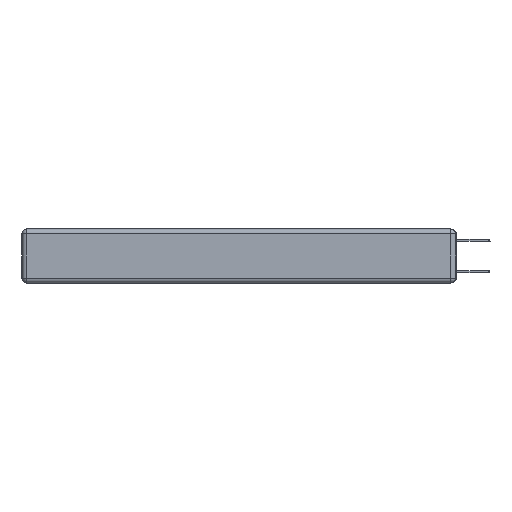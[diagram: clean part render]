
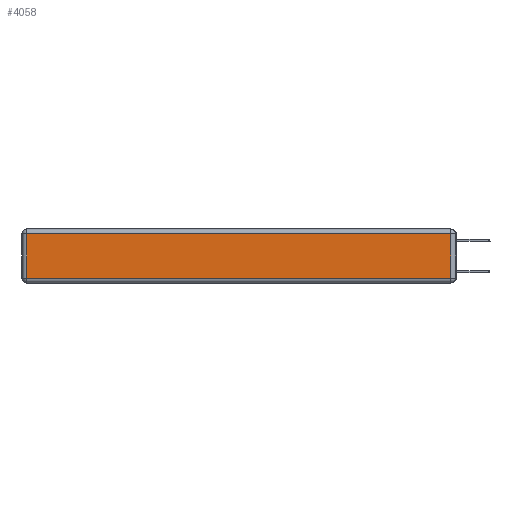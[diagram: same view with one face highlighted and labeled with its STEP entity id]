
A CAD part, left-side view. The second image highlights one B-rep face of the part: STEP entity #4058.
In plain terms, the highlighted planar face has unit normal (-1, 0, 0).
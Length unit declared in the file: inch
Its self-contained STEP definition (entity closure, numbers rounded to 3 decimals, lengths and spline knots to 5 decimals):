
#633 = VERTEX_POINT ( 'NONE', #15095 ) ;
#755 = PLANE ( 'NONE',  #25407 ) ;
#1755 = VERTEX_POINT ( 'NONE', #6588 ) ;
#2178 = ORIENTED_EDGE ( 'NONE', *, *, #19815, .T. ) ;
#2660 = EDGE_CURVE ( 'NONE', #22898, #25426, #4708, .T. ) ;
#3557 = VECTOR ( 'NONE', #8804, 39.37008 ) ;
#4058 = ADVANCED_FACE ( 'NONE', ( #20680 ), #755, .T. ) ;
#4284 = CARTESIAN_POINT ( 'NONE',  ( 0., 0., -0.343 ) ) ;
#4708 = LINE ( 'NONE', #10256, #4742 ) ;
#4742 = VECTOR ( 'NONE', #12332, 39.37008 ) ;
#4829 = VECTOR ( 'NONE', #8323, 39.37008 ) ;
#5794 = LINE ( 'NONE', #19991, #19730 ) ;
#6588 = CARTESIAN_POINT ( 'NONE',  ( 0., 2.72, -0.03 ) ) ;
#6916 = ORIENTED_EDGE ( 'NONE', *, *, #22636, .T. ) ;
#7778 = LINE ( 'NONE', #23567, #3557 ) ;
#8323 = DIRECTION ( 'NONE',  ( 0., 1., 0. ) ) ;
#8442 = CARTESIAN_POINT ( 'NONE',  ( 0., 2.75, -0.03 ) ) ;
#8804 = DIRECTION ( 'NONE',  ( 0., 0., -1. ) ) ;
#10256 = CARTESIAN_POINT ( 'NONE',  ( 0., 0., -0.313 ) ) ;
#10492 = LINE ( 'NONE', #8442, #4829 ) ;
#11181 = ORIENTED_EDGE ( 'NONE', *, *, #17648, .T. ) ;
#12332 = DIRECTION ( 'NONE',  ( 0., -1., 0. ) ) ;
#13031 = DIRECTION ( 'NONE',  ( 0., 0., 1. ) ) ;
#14713 = DIRECTION ( 'NONE',  ( -1., 0., 0. ) ) ;
#15095 = CARTESIAN_POINT ( 'NONE',  ( 0., 0.03, -0.03 ) ) ;
#17648 = EDGE_CURVE ( 'NONE', #1755, #22898, #7778, .T. ) ;
#19730 = VECTOR ( 'NONE', #19871, 39.37008 ) ;
#19815 = EDGE_CURVE ( 'NONE', #25426, #633, #5794, .T. ) ;
#19871 = DIRECTION ( 'NONE',  ( 0., 0., 1. ) ) ;
#19909 = EDGE_LOOP ( 'NONE', ( #21451, #2178, #6916, #11181 ) ) ;
#19991 = CARTESIAN_POINT ( 'NONE',  ( 0., 0.03, -0.343 ) ) ;
#20164 = CARTESIAN_POINT ( 'NONE',  ( 0., 0.03, -0.313 ) ) ;
#20680 = FACE_OUTER_BOUND ( 'NONE', #19909, .T. ) ;
#21451 = ORIENTED_EDGE ( 'NONE', *, *, #2660, .T. ) ;
#22636 = EDGE_CURVE ( 'NONE', #633, #1755, #10492, .T. ) ;
#22898 = VERTEX_POINT ( 'NONE', #25481 ) ;
#23567 = CARTESIAN_POINT ( 'NONE',  ( 0., 2.72, -0.343 ) ) ;
#25407 = AXIS2_PLACEMENT_3D ( 'NONE', #4284, #14713, #13031 ) ;
#25426 = VERTEX_POINT ( 'NONE', #20164 ) ;
#25481 = CARTESIAN_POINT ( 'NONE',  ( 0., 2.72, -0.313 ) ) ;
